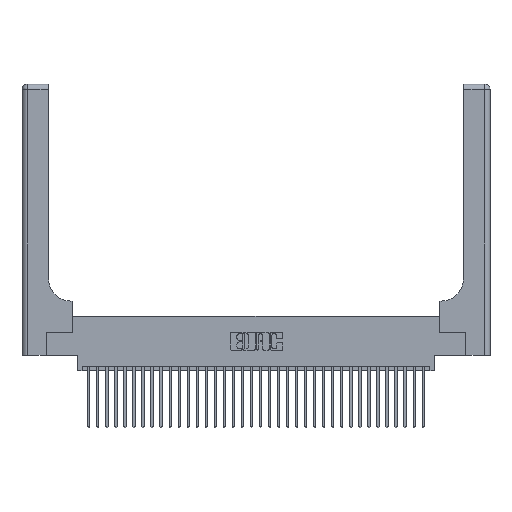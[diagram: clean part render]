
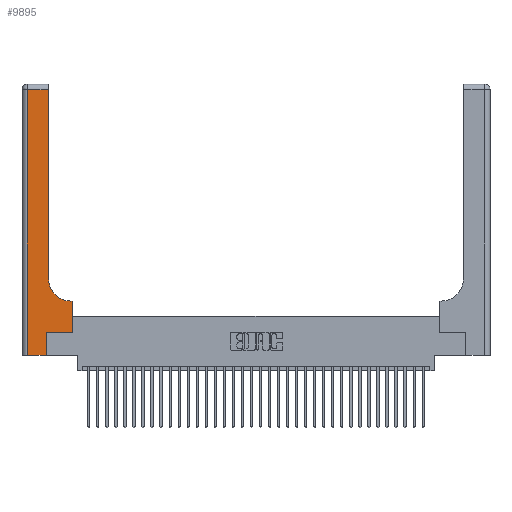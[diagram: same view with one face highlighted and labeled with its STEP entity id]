
A CAD part, top view. The second image highlights one B-rep face of the part: STEP entity #9895.
In plain terms, the highlighted planar face has unit normal (0, 0, 1).
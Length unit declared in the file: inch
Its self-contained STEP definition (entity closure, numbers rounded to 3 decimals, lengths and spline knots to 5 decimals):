
#570 = CARTESIAN_POINT ( 'NONE',  ( 0.5585, 0.25, 0.37 ) ) ;
#703 = EDGE_CURVE ( 'NONE', #12728, #21733, #21700, .T. ) ;
#1135 = ORIENTED_EDGE ( 'NONE', *, *, #18343, .T. ) ;
#1171 = ORIENTED_EDGE ( 'NONE', *, *, #28954, .T. ) ;
#2366 = ORIENTED_EDGE ( 'NONE', *, *, #2791, .T. ) ;
#2645 = CARTESIAN_POINT ( 'NONE',  ( 0.2915, 0.85, 0.37 ) ) ;
#2784 = CARTESIAN_POINT ( 'NONE',  ( 0.5585, 0.25, 0.37 ) ) ;
#2791 = EDGE_CURVE ( 'NONE', #35246, #15077, #24179, .T. ) ;
#3451 = VERTEX_POINT ( 'NONE', #14563 ) ;
#3699 = AXIS2_PLACEMENT_3D ( 'NONE', #21085, #4496, #23849 ) ;
#3784 = ORIENTED_EDGE ( 'NONE', *, *, #17757, .T. ) ;
#4496 = DIRECTION ( 'NONE',  ( 0., 0., -1. ) ) ;
#5471 = ORIENTED_EDGE ( 'NONE', *, *, #17882, .T. ) ;
#6348 = ORIENTED_EDGE ( 'NONE', *, *, #19923, .T. ) ;
#6613 = CARTESIAN_POINT ( 'NONE',  ( 0., 0., 0.37 ) ) ;
#6788 = CARTESIAN_POINT ( 'NONE',  ( 0.06, 3., 0.37 ) ) ;
#6950 = DIRECTION ( 'NONE',  ( 0., 0., -1. ) ) ;
#7834 = VECTOR ( 'NONE', #20447, 39.37008 ) ;
#8489 = AXIS2_PLACEMENT_3D ( 'NONE', #15264, #6950, #26277 ) ;
#9117 = CARTESIAN_POINT ( 'NONE',  ( 0.5585, 0.6, 0.37 ) ) ;
#9120 = VECTOR ( 'NONE', #12851, 39.37008 ) ;
#9702 = FACE_OUTER_BOUND ( 'NONE', #31656, .T. ) ;
#9895 = ADVANCED_FACE ( 'NONE', ( #9702 ), #34388, .F. ) ;
#10915 = VERTEX_POINT ( 'NONE', #570 ) ;
#12257 = DIRECTION ( 'NONE',  ( -1., 0., 0. ) ) ;
#12728 = VERTEX_POINT ( 'NONE', #18720 ) ;
#12851 = DIRECTION ( 'NONE',  ( 1., 0., 0. ) ) ;
#13313 = CARTESIAN_POINT ( 'NONE',  ( 0.2915, 2.94, 0.37 ) ) ;
#13374 = DIRECTION ( 'NONE',  ( 0., 1., 0. ) ) ;
#13551 = LINE ( 'NONE', #29865, #34556 ) ;
#14563 = CARTESIAN_POINT ( 'NONE',  ( 0.269, 0.25, 0.37 ) ) ;
#14817 = CARTESIAN_POINT ( 'NONE',  ( 0.2915, 0.6, 0.37 ) ) ;
#15077 = VERTEX_POINT ( 'NONE', #2645 ) ;
#15264 = CARTESIAN_POINT ( 'NONE',  ( 0., 3., 0.37 ) ) ;
#15277 = LINE ( 'NONE', #14817, #7834 ) ;
#16554 = LINE ( 'NONE', #21035, #9120 ) ;
#17529 = VECTOR ( 'NONE', #28728, 39.37008 ) ;
#17757 = EDGE_CURVE ( 'NONE', #33911, #3451, #13551, .T. ) ;
#17882 = EDGE_CURVE ( 'NONE', #10915, #27834, #23868, .T. ) ;
#18146 = EDGE_CURVE ( 'NONE', #27834, #35246, #15277, .T. ) ;
#18343 = EDGE_CURVE ( 'NONE', #3451, #10915, #16554, .T. ) ;
#18720 = CARTESIAN_POINT ( 'NONE',  ( 0.06, 2.94, 0.37 ) ) ;
#19923 = EDGE_CURVE ( 'NONE', #27499, #12728, #31071, .T. ) ;
#20141 = CARTESIAN_POINT ( 'NONE',  ( 0.2915, 3., 0.37 ) ) ;
#20447 = DIRECTION ( 'NONE',  ( -1., 0., 0. ) ) ;
#21035 = CARTESIAN_POINT ( 'NONE',  ( 0.269, 0.25, 0.37 ) ) ;
#21085 = CARTESIAN_POINT ( 'NONE',  ( 0.5415, 0.85, 0.37 ) ) ;
#21229 = CARTESIAN_POINT ( 'NONE',  ( 0.5415, 0.6, 0.37 ) ) ;
#21700 = LINE ( 'NONE', #6788, #22165 ) ;
#21733 = VERTEX_POINT ( 'NONE', #32047 ) ;
#21840 = LINE ( 'NONE', #20141, #34670 ) ;
#22165 = VECTOR ( 'NONE', #26121, 39.37008 ) ;
#22894 = DIRECTION ( 'NONE',  ( 0., 1., 0. ) ) ;
#23768 = VECTOR ( 'NONE', #12257, 39.37008 ) ;
#23849 = DIRECTION ( 'NONE',  ( 1., 0., 0. ) ) ;
#23868 = LINE ( 'NONE', #2784, #30328 ) ;
#24179 = CIRCLE ( 'NONE', #3699, 0.25 ) ;
#25679 = LINE ( 'NONE', #6613, #17529 ) ;
#25729 = CARTESIAN_POINT ( 'NONE',  ( 0., 2.94, 0.37 ) ) ;
#25764 = EDGE_CURVE ( 'NONE', #15077, #27499, #21840, .T. ) ;
#26121 = DIRECTION ( 'NONE',  ( 0., -1., 0. ) ) ;
#26277 = DIRECTION ( 'NONE',  ( -1., 0., 0. ) ) ;
#27499 = VERTEX_POINT ( 'NONE', #13313 ) ;
#27834 = VERTEX_POINT ( 'NONE', #9117 ) ;
#28049 = CARTESIAN_POINT ( 'NONE',  ( 0.269, 0., 0.37 ) ) ;
#28728 = DIRECTION ( 'NONE',  ( 1., 0., 0. ) ) ;
#28858 = ORIENTED_EDGE ( 'NONE', *, *, #703, .T. ) ;
#28954 = EDGE_CURVE ( 'NONE', #21733, #33911, #25679, .T. ) ;
#29865 = CARTESIAN_POINT ( 'NONE',  ( 0.269, 0., 0.37 ) ) ;
#30328 = VECTOR ( 'NONE', #32922, 39.37008 ) ;
#30547 = ORIENTED_EDGE ( 'NONE', *, *, #25764, .T. ) ;
#31071 = LINE ( 'NONE', #25729, #23768 ) ;
#31656 = EDGE_LOOP ( 'NONE', ( #30547, #6348, #28858, #1171, #3784, #1135, #5471, #35620, #2366 ) ) ;
#32047 = CARTESIAN_POINT ( 'NONE',  ( 0.06, 0., 0.37 ) ) ;
#32922 = DIRECTION ( 'NONE',  ( 0., 1., 0. ) ) ;
#33911 = VERTEX_POINT ( 'NONE', #28049 ) ;
#34388 = PLANE ( 'NONE',  #8489 ) ;
#34556 = VECTOR ( 'NONE', #13374, 39.37008 ) ;
#34670 = VECTOR ( 'NONE', #22894, 39.37008 ) ;
#35246 = VERTEX_POINT ( 'NONE', #21229 ) ;
#35620 = ORIENTED_EDGE ( 'NONE', *, *, #18146, .T. ) ;
